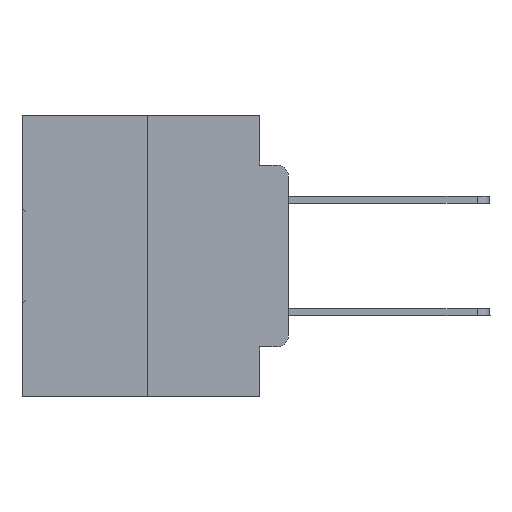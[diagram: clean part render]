
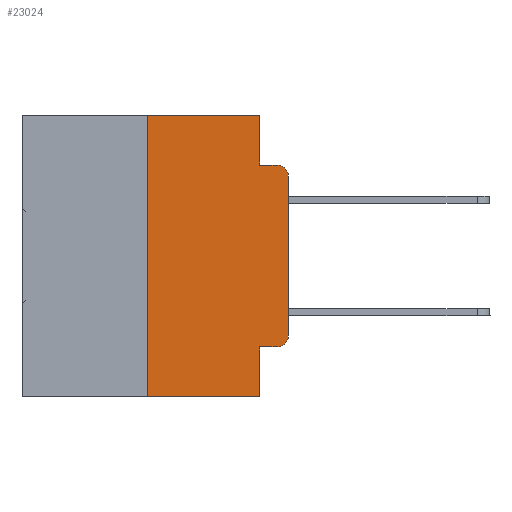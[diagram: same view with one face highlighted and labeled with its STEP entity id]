
A CAD part, left-side view. The second image highlights one B-rep face of the part: STEP entity #23024.
In plain terms, the highlighted planar face has unit normal (-1, 0, 0).
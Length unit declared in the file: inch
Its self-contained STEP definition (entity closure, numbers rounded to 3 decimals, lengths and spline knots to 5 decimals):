
#38 = DIRECTION ( 'NONE',  ( 1., 0., 0. ) ) ;
#50 = CARTESIAN_POINT ( 'NONE',  ( 0., 0.473, -0.5 ) ) ;
#151 = DIRECTION ( 'NONE',  ( 0., 0., -1. ) ) ;
#155 = CARTESIAN_POINT ( 'NONE',  ( 0., 0.051, 0. ) ) ;
#244 = DIRECTION ( 'NONE',  ( 0., 0., -1. ) ) ;
#538 = CARTESIAN_POINT ( 'NONE',  ( 0., 0.051, 0. ) ) ;
#854 = LINE ( 'NONE', #4738, #17702 ) ;
#1070 = CARTESIAN_POINT ( 'NONE',  ( 0., 0.02, -0.3915 ) ) ;
#1191 = DIRECTION ( 'NONE',  ( 0., 0., -1. ) ) ;
#1267 = ORIENTED_EDGE ( 'NONE', *, *, #31962, .T. ) ;
#1528 = ORIENTED_EDGE ( 'NONE', *, *, #19468, .F. ) ;
#2268 = EDGE_CURVE ( 'NONE', #25037, #6608, #21817, .T. ) ;
#2992 = LINE ( 'NONE', #10245, #31515 ) ;
#3858 = CIRCLE ( 'NONE', #20784, 0.02 ) ;
#4738 = CARTESIAN_POINT ( 'NONE',  ( 0., 0.473, 0. ) ) ;
#5184 = VERTEX_POINT ( 'NONE', #19929 ) ;
#5896 = EDGE_CURVE ( 'NONE', #22087, #31372, #13248, .T. ) ;
#6608 = VERTEX_POINT ( 'NONE', #14362 ) ;
#6988 = ORIENTED_EDGE ( 'NONE', *, *, #19936, .T. ) ;
#8173 = CARTESIAN_POINT ( 'NONE',  ( 0., 0., -0.1085 ) ) ;
#8823 = DIRECTION ( 'NONE',  ( 0., 0., -1. ) ) ;
#9361 = DIRECTION ( 'NONE',  ( 0., -1., 0. ) ) ;
#9984 = CARTESIAN_POINT ( 'NONE',  ( 0., 0.02, -0.0885 ) ) ;
#10245 = CARTESIAN_POINT ( 'NONE',  ( 0., 0.051, -0.0885 ) ) ;
#10451 = EDGE_CURVE ( 'NONE', #25037, #12175, #18532, .T. ) ;
#10472 = DIRECTION ( 'NONE',  ( 0., -1., 0. ) ) ;
#10488 = EDGE_CURVE ( 'NONE', #12175, #25067, #854, .T. ) ;
#10516 = VERTEX_POINT ( 'NONE', #9984 ) ;
#10840 = DIRECTION ( 'NONE',  ( 0., -1., 0. ) ) ;
#11135 = VECTOR ( 'NONE', #244, 39.37008 ) ;
#11187 = CARTESIAN_POINT ( 'NONE',  ( 0., 0.25, -0.5 ) ) ;
#11777 = VERTEX_POINT ( 'NONE', #8173 ) ;
#11988 = DIRECTION ( 'NONE',  ( 0., 0., -1. ) ) ;
#12175 = VERTEX_POINT ( 'NONE', #18401 ) ;
#12731 = CARTESIAN_POINT ( 'NONE',  ( 0., 0.25, 0. ) ) ;
#13248 = LINE ( 'NONE', #30837, #33742 ) ;
#14362 = CARTESIAN_POINT ( 'NONE',  ( 0., 0.051, -0.5 ) ) ;
#14730 = DIRECTION ( 'NONE',  ( -1., 0., 0. ) ) ;
#14862 = ORIENTED_EDGE ( 'NONE', *, *, #34025, .F. ) ;
#15961 = CARTESIAN_POINT ( 'NONE',  ( 0., 0., 0. ) ) ;
#15991 = CARTESIAN_POINT ( 'NONE',  ( 0., 0.051, -0.0885 ) ) ;
#16447 = VECTOR ( 'NONE', #20563, 39.37008 ) ;
#17702 = VECTOR ( 'NONE', #23479, 39.37008 ) ;
#18401 = CARTESIAN_POINT ( 'NONE',  ( 0., 0.25, 0. ) ) ;
#18503 = FACE_OUTER_BOUND ( 'NONE', #24049, .T. ) ;
#18532 = LINE ( 'NONE', #12731, #16447 ) ;
#18860 = ORIENTED_EDGE ( 'NONE', *, *, #10451, .F. ) ;
#19468 = EDGE_CURVE ( 'NONE', #23702, #10516, #2992, .T. ) ;
#19929 = CARTESIAN_POINT ( 'NONE',  ( 0., 0., -0.3915 ) ) ;
#19936 = EDGE_CURVE ( 'NONE', #11777, #10516, #22710, .T. ) ;
#20563 = DIRECTION ( 'NONE',  ( 0., 0., 1. ) ) ;
#20784 = AXIS2_PLACEMENT_3D ( 'NONE', #1070, #14730, #1191 ) ;
#21373 = ORIENTED_EDGE ( 'NONE', *, *, #10488, .F. ) ;
#21689 = CARTESIAN_POINT ( 'NONE',  ( 0., 0.051, -0.4115 ) ) ;
#21817 = LINE ( 'NONE', #50, #24798 ) ;
#22087 = VERTEX_POINT ( 'NONE', #21689 ) ;
#22710 = CIRCLE ( 'NONE', #29942, 0.02 ) ;
#23024 = ADVANCED_FACE ( 'NONE', ( #18503 ), #27055, .F. ) ;
#23162 = LINE ( 'NONE', #15961, #30690 ) ;
#23479 = DIRECTION ( 'NONE',  ( 0., -1., 0. ) ) ;
#23702 = VERTEX_POINT ( 'NONE', #15991 ) ;
#24049 = EDGE_LOOP ( 'NONE', ( #1267, #6988, #1528, #14862, #21373, #18860, #27307, #32272, #32683, #31974 ) ) ;
#24798 = VECTOR ( 'NONE', #10840, 39.37008 ) ;
#25037 = VERTEX_POINT ( 'NONE', #11187 ) ;
#25067 = VERTEX_POINT ( 'NONE', #155 ) ;
#25484 = DIRECTION ( 'NONE',  ( -1., 0., 0. ) ) ;
#26272 = LINE ( 'NONE', #32816, #11135 ) ;
#26326 = CARTESIAN_POINT ( 'NONE',  ( 0., 0.02, -0.4115 ) ) ;
#26732 = EDGE_CURVE ( 'NONE', #22087, #6608, #26272, .T. ) ;
#26919 = AXIS2_PLACEMENT_3D ( 'NONE', #32039, #38, #151 ) ;
#27055 = PLANE ( 'NONE',  #26919 ) ;
#27307 = ORIENTED_EDGE ( 'NONE', *, *, #2268, .T. ) ;
#27625 = LINE ( 'NONE', #538, #31792 ) ;
#29942 = AXIS2_PLACEMENT_3D ( 'NONE', #33499, #25484, #11988 ) ;
#30690 = VECTOR ( 'NONE', #34623, 39.37008 ) ;
#30837 = CARTESIAN_POINT ( 'NONE',  ( 0., 0.051, -0.4115 ) ) ;
#31035 = EDGE_CURVE ( 'NONE', #31372, #5184, #3858, .T. ) ;
#31372 = VERTEX_POINT ( 'NONE', #26326 ) ;
#31515 = VECTOR ( 'NONE', #10472, 39.37008 ) ;
#31792 = VECTOR ( 'NONE', #8823, 39.37008 ) ;
#31962 = EDGE_CURVE ( 'NONE', #5184, #11777, #23162, .T. ) ;
#31974 = ORIENTED_EDGE ( 'NONE', *, *, #31035, .T. ) ;
#32039 = CARTESIAN_POINT ( 'NONE',  ( 0., 0.473, 0. ) ) ;
#32272 = ORIENTED_EDGE ( 'NONE', *, *, #26732, .F. ) ;
#32683 = ORIENTED_EDGE ( 'NONE', *, *, #5896, .T. ) ;
#32816 = CARTESIAN_POINT ( 'NONE',  ( 0., 0.051, 0. ) ) ;
#33499 = CARTESIAN_POINT ( 'NONE',  ( 0., 0.02, -0.1085 ) ) ;
#33742 = VECTOR ( 'NONE', #9361, 39.37008 ) ;
#34025 = EDGE_CURVE ( 'NONE', #25067, #23702, #27625, .T. ) ;
#34623 = DIRECTION ( 'NONE',  ( 0., 0., 1. ) ) ;
